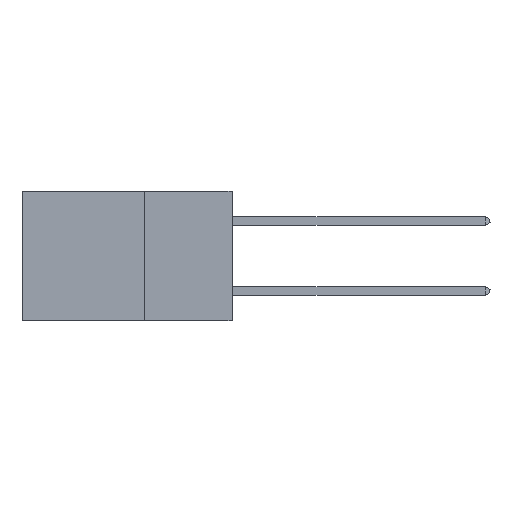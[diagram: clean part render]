
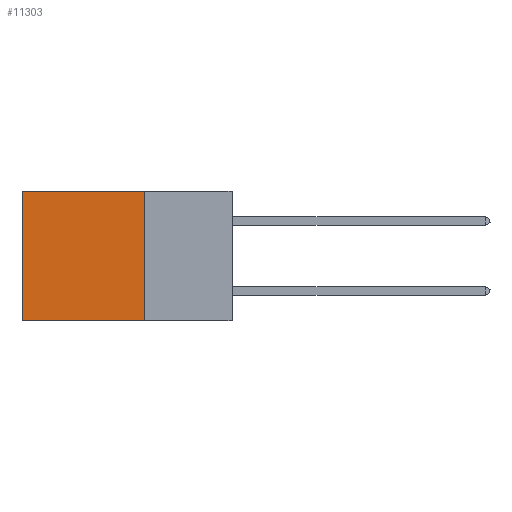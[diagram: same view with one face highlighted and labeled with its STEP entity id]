
A CAD part, left-side view. The second image highlights one B-rep face of the part: STEP entity #11303.
In plain terms, the highlighted planar face has unit normal (-1, 0, 0).
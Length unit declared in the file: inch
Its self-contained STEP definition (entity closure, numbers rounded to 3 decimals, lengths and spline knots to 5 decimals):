
#1091 = CARTESIAN_POINT ( 'NONE',  ( 0.2875, 0.6, 0. ) ) ;
#2326 = DIRECTION ( 'NONE',  ( 0., 1., 0. ) ) ;
#2828 = CARTESIAN_POINT ( 'NONE',  ( 0.2875, 0.25, 0. ) ) ;
#3175 = VECTOR ( 'NONE', #28858, 39.37008 ) ;
#3191 = EDGE_CURVE ( 'NONE', #7927, #27761, #31556, .T. ) ;
#3907 = DIRECTION ( 'NONE',  ( 0., 0., -1. ) ) ;
#4201 = CARTESIAN_POINT ( 'NONE',  ( 0.2875, 0.25, 0. ) ) ;
#5404 = PLANE ( 'NONE',  #11948 ) ;
#7927 = VERTEX_POINT ( 'NONE', #19822 ) ;
#9483 = ORIENTED_EDGE ( 'NONE', *, *, #28341, .T. ) ;
#10580 = DIRECTION ( 'NONE',  ( 0., 0., -1. ) ) ;
#10825 = ORIENTED_EDGE ( 'NONE', *, *, #3191, .F. ) ;
#11063 = CARTESIAN_POINT ( 'NONE',  ( 0.2875, 0.25, -0.37 ) ) ;
#11303 = ADVANCED_FACE ( 'NONE', ( #11460 ), #5404, .F. ) ;
#11460 = FACE_OUTER_BOUND ( 'NONE', #19574, .T. ) ;
#11948 = AXIS2_PLACEMENT_3D ( 'NONE', #12751, #20564, #10580 ) ;
#12751 = CARTESIAN_POINT ( 'NONE',  ( 0.2875, 0.25, 0. ) ) ;
#13175 = CARTESIAN_POINT ( 'NONE',  ( 0.2875, 0.6, 0. ) ) ;
#13567 = DIRECTION ( 'NONE',  ( 0., 1., 0. ) ) ;
#16855 = VERTEX_POINT ( 'NONE', #13175 ) ;
#17212 = ORIENTED_EDGE ( 'NONE', *, *, #31805, .T. ) ;
#17866 = EDGE_CURVE ( 'NONE', #30562, #7927, #18942, .T. ) ;
#18854 = ORIENTED_EDGE ( 'NONE', *, *, #17866, .F. ) ;
#18942 = LINE ( 'NONE', #2828, #3175 ) ;
#19574 = EDGE_LOOP ( 'NONE', ( #17212, #10825, #18854, #9483 ) ) ;
#19822 = CARTESIAN_POINT ( 'NONE',  ( 0.2875, 0.25, -0.37 ) ) ;
#20564 = DIRECTION ( 'NONE',  ( 1., 0., 0. ) ) ;
#22886 = VECTOR ( 'NONE', #3907, 39.37008 ) ;
#23012 = CARTESIAN_POINT ( 'NONE',  ( 0.2875, 0.25, 0. ) ) ;
#25546 = VECTOR ( 'NONE', #2326, 39.37008 ) ;
#27761 = VERTEX_POINT ( 'NONE', #28482 ) ;
#27945 = VECTOR ( 'NONE', #13567, 39.37008 ) ;
#28341 = EDGE_CURVE ( 'NONE', #30562, #16855, #32853, .T. ) ;
#28482 = CARTESIAN_POINT ( 'NONE',  ( 0.2875, 0.6, -0.37 ) ) ;
#28858 = DIRECTION ( 'NONE',  ( 0., 0., -1. ) ) ;
#29776 = LINE ( 'NONE', #1091, #22886 ) ;
#30562 = VERTEX_POINT ( 'NONE', #4201 ) ;
#31556 = LINE ( 'NONE', #11063, #27945 ) ;
#31805 = EDGE_CURVE ( 'NONE', #16855, #27761, #29776, .T. ) ;
#32853 = LINE ( 'NONE', #23012, #25546 ) ;
